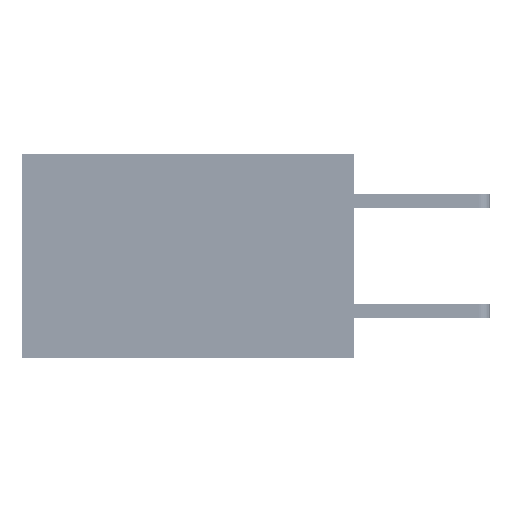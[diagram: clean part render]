
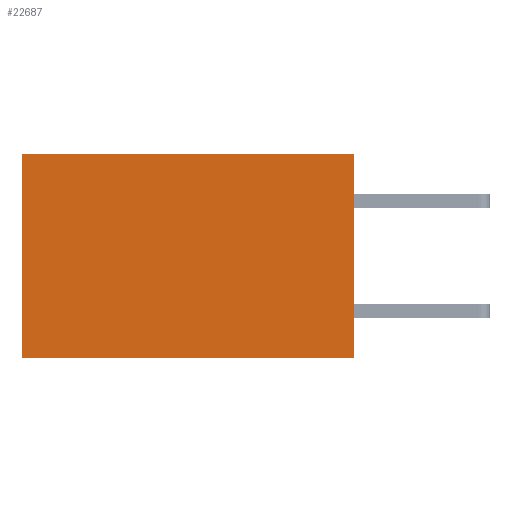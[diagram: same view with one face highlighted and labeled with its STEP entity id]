
A CAD part, left-side view. The second image highlights one B-rep face of the part: STEP entity #22687.
In plain terms, the highlighted planar face has unit normal (-1, 0, 0).
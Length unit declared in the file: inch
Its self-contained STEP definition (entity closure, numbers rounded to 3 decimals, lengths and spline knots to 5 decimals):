
#2124 = VECTOR ( 'NONE', #31526, 39.37008 ) ;
#2528 = DIRECTION ( 'NONE',  ( 1., 0., 0. ) ) ;
#3088 = AXIS2_PLACEMENT_3D ( 'NONE', #11458, #2528, #14595 ) ;
#4668 = CARTESIAN_POINT ( 'NONE',  ( 0.2875, 0., 0. ) ) ;
#6365 = LINE ( 'NONE', #33459, #2124 ) ;
#6773 = LINE ( 'NONE', #4668, #32898 ) ;
#7643 = ORIENTED_EDGE ( 'NONE', *, *, #19856, .F. ) ;
#9183 = ORIENTED_EDGE ( 'NONE', *, *, #27421, .F. ) ;
#9662 = VERTEX_POINT ( 'NONE', #20859 ) ;
#11458 = CARTESIAN_POINT ( 'NONE',  ( 0.2875, 0., 0. ) ) ;
#14023 = CARTESIAN_POINT ( 'NONE',  ( 0.2875, 0.6, -0.37 ) ) ;
#14595 = DIRECTION ( 'NONE',  ( 0., 0., -1. ) ) ;
#15298 = CARTESIAN_POINT ( 'NONE',  ( 0.2875, 0., -0.37 ) ) ;
#15832 = LINE ( 'NONE', #24316, #17803 ) ;
#17803 = VECTOR ( 'NONE', #19025, 39.37008 ) ;
#18007 = EDGE_CURVE ( 'NONE', #23689, #37353, #6365, .T. ) ;
#19025 = DIRECTION ( 'NONE',  ( 0., 1., 0. ) ) ;
#19856 = EDGE_CURVE ( 'NONE', #26365, #37353, #30740, .T. ) ;
#20859 = CARTESIAN_POINT ( 'NONE',  ( 0.2875, 0., 0. ) ) ;
#22687 = ADVANCED_FACE ( 'NONE', ( #36549 ), #29996, .F. ) ;
#23689 = VERTEX_POINT ( 'NONE', #26253 ) ;
#24033 = EDGE_CURVE ( 'NONE', #9662, #23689, #15832, .T. ) ;
#24316 = CARTESIAN_POINT ( 'NONE',  ( 0.2875, 0., 0. ) ) ;
#26201 = CARTESIAN_POINT ( 'NONE',  ( 0.2875, 0., -0.37 ) ) ;
#26253 = CARTESIAN_POINT ( 'NONE',  ( 0.2875, 0.6, 0. ) ) ;
#26365 = VERTEX_POINT ( 'NONE', #15298 ) ;
#27421 = EDGE_CURVE ( 'NONE', #9662, #26365, #6773, .T. ) ;
#29996 = PLANE ( 'NONE',  #3088 ) ;
#30740 = LINE ( 'NONE', #26201, #33640 ) ;
#31526 = DIRECTION ( 'NONE',  ( 0., 0., -1. ) ) ;
#31546 = EDGE_LOOP ( 'NONE', ( #33470, #7643, #9183, #38155 ) ) ;
#32420 = DIRECTION ( 'NONE',  ( 0., 0., -1. ) ) ;
#32898 = VECTOR ( 'NONE', #32420, 39.37008 ) ;
#33459 = CARTESIAN_POINT ( 'NONE',  ( 0.2875, 0.6, 0. ) ) ;
#33470 = ORIENTED_EDGE ( 'NONE', *, *, #18007, .T. ) ;
#33640 = VECTOR ( 'NONE', #38589, 39.37008 ) ;
#36549 = FACE_OUTER_BOUND ( 'NONE', #31546, .T. ) ;
#37353 = VERTEX_POINT ( 'NONE', #14023 ) ;
#38155 = ORIENTED_EDGE ( 'NONE', *, *, #24033, .T. ) ;
#38589 = DIRECTION ( 'NONE',  ( 0., 1., 0. ) ) ;
